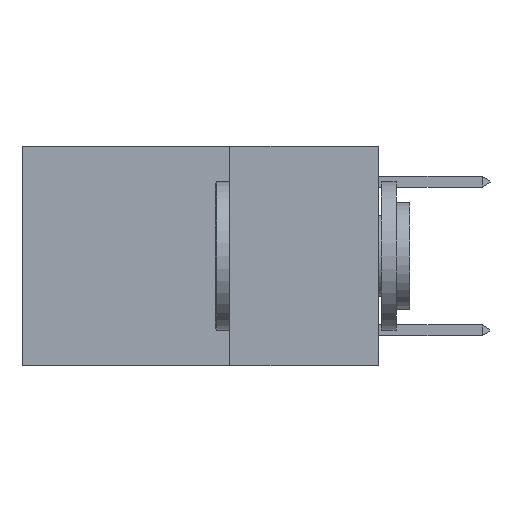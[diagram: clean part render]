
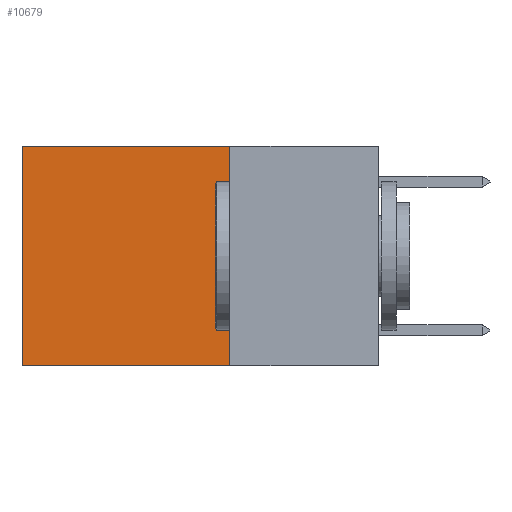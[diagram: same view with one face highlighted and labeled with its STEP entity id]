
A CAD part, left-side view. The second image highlights one B-rep face of the part: STEP entity #10679.
In plain terms, the highlighted planar face has unit normal (-1, 0, 0).
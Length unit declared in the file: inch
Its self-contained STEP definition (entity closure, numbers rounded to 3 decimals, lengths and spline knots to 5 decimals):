
#224 = CARTESIAN_POINT ( 'NONE',  ( 0.2625, 0.25, -0.37 ) ) ;
#515 = CARTESIAN_POINT ( 'NONE',  ( 0.2625, 0.25, -0.37 ) ) ;
#610 = EDGE_CURVE ( 'NONE', #17197, #12454, #5114, .T. ) ;
#1095 = ORIENTED_EDGE ( 'NONE', *, *, #610, .F. ) ;
#1616 = VERTEX_POINT ( 'NONE', #17319 ) ;
#1736 = LINE ( 'NONE', #11333, #16999 ) ;
#2255 = DIRECTION ( 'NONE',  ( 0., 0., -1. ) ) ;
#4121 = ORIENTED_EDGE ( 'NONE', *, *, #24561, .T. ) ;
#4424 = EDGE_LOOP ( 'NONE', ( #21371, #12096, #1095, #4121 ) ) ;
#4564 = AXIS2_PLACEMENT_3D ( 'NONE', #20055, #23802, #18029 ) ;
#4898 = VECTOR ( 'NONE', #10508, 39.37008 ) ;
#5114 = LINE ( 'NONE', #23699, #9098 ) ;
#6569 = CARTESIAN_POINT ( 'NONE',  ( 0.2625, 0.6, 0. ) ) ;
#6744 = LINE ( 'NONE', #515, #4898 ) ;
#7075 = CARTESIAN_POINT ( 'NONE',  ( 0.2625, 0.25, 0. ) ) ;
#9098 = VECTOR ( 'NONE', #12074, 39.37008 ) ;
#10508 = DIRECTION ( 'NONE',  ( 0., 1., 0. ) ) ;
#10679 = ADVANCED_FACE ( 'NONE', ( #21865 ), #17945, .F. ) ;
#11294 = EDGE_CURVE ( 'NONE', #12454, #1616, #6744, .T. ) ;
#11333 = CARTESIAN_POINT ( 'NONE',  ( 0.2625, 0.25, 0. ) ) ;
#11731 = VERTEX_POINT ( 'NONE', #6569 ) ;
#12074 = DIRECTION ( 'NONE',  ( 0., 0., -1. ) ) ;
#12096 = ORIENTED_EDGE ( 'NONE', *, *, #11294, .F. ) ;
#12454 = VERTEX_POINT ( 'NONE', #224 ) ;
#15697 = VECTOR ( 'NONE', #2255, 39.37008 ) ;
#16999 = VECTOR ( 'NONE', #19551, 39.37008 ) ;
#17197 = VERTEX_POINT ( 'NONE', #7075 ) ;
#17319 = CARTESIAN_POINT ( 'NONE',  ( 0.2625, 0.6, -0.37 ) ) ;
#17945 = PLANE ( 'NONE',  #4564 ) ;
#18029 = DIRECTION ( 'NONE',  ( 0., 0., -1. ) ) ;
#19551 = DIRECTION ( 'NONE',  ( 0., 1., 0. ) ) ;
#20055 = CARTESIAN_POINT ( 'NONE',  ( 0.2625, 0.25, 0. ) ) ;
#20220 = LINE ( 'NONE', #21761, #15697 ) ;
#21371 = ORIENTED_EDGE ( 'NONE', *, *, #22563, .T. ) ;
#21761 = CARTESIAN_POINT ( 'NONE',  ( 0.2625, 0.6, 0. ) ) ;
#21865 = FACE_OUTER_BOUND ( 'NONE', #4424, .T. ) ;
#22563 = EDGE_CURVE ( 'NONE', #11731, #1616, #20220, .T. ) ;
#23699 = CARTESIAN_POINT ( 'NONE',  ( 0.2625, 0.25, 0. ) ) ;
#23802 = DIRECTION ( 'NONE',  ( 1., 0., 0. ) ) ;
#24561 = EDGE_CURVE ( 'NONE', #17197, #11731, #1736, .T. ) ;
